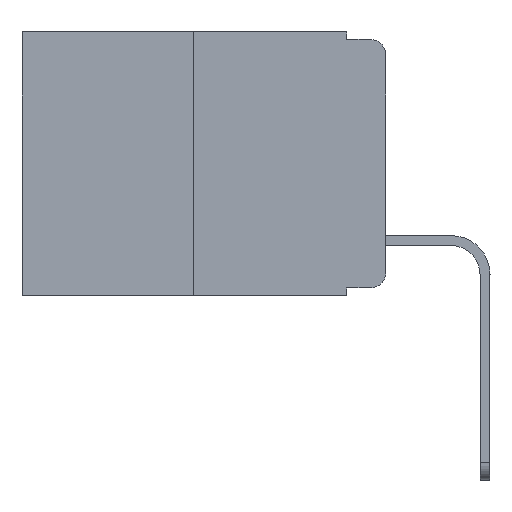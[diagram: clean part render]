
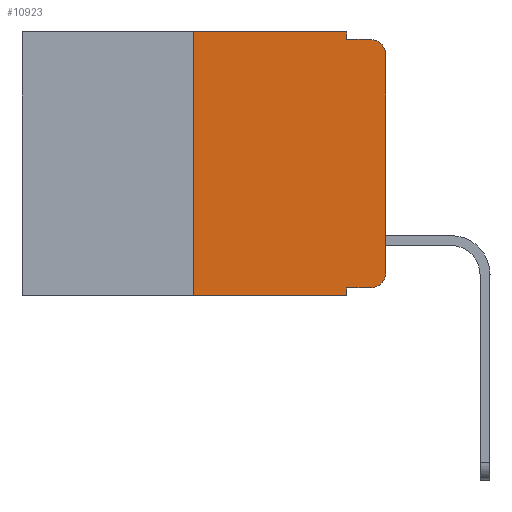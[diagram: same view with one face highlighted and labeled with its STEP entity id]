
A CAD part, left-side view. The second image highlights one B-rep face of the part: STEP entity #10923.
In plain terms, the highlighted planar face has unit normal (-1, 0, 0).
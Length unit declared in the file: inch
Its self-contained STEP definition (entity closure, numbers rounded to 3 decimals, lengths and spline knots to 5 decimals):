
#735 = AXIS2_PLACEMENT_3D ( 'NONE', #8578, #4028, #10306 ) ;
#1139 = ORIENTED_EDGE ( 'NONE', *, *, #16479, .F. ) ;
#1734 = VERTEX_POINT ( 'NONE', #15935 ) ;
#1859 = ORIENTED_EDGE ( 'NONE', *, *, #16016, .T. ) ;
#1916 = VECTOR ( 'NONE', #7416, 39.37008 ) ;
#2189 = EDGE_CURVE ( 'NONE', #13208, #11674, #11388, .T. ) ;
#2305 = VERTEX_POINT ( 'NONE', #10817 ) ;
#2534 = CARTESIAN_POINT ( 'NONE',  ( 0., 0.051, 0. ) ) ;
#2593 = CARTESIAN_POINT ( 'NONE',  ( 0., 0., -0.313 ) ) ;
#2648 = AXIS2_PLACEMENT_3D ( 'NONE', #5903, #4383, #7565 ) ;
#2926 = DIRECTION ( 'NONE',  ( 0., 0., -1. ) ) ;
#3054 = VECTOR ( 'NONE', #14408, 39.37008 ) ;
#3266 = ORIENTED_EDGE ( 'NONE', *, *, #9544, .F. ) ;
#3595 = LINE ( 'NONE', #6675, #12977 ) ;
#4028 = DIRECTION ( 'NONE',  ( -1., 0., 0. ) ) ;
#4291 = DIRECTION ( 'NONE',  ( 0., 0., 1. ) ) ;
#4344 = DIRECTION ( 'NONE',  ( 0., 0., 1. ) ) ;
#4383 = DIRECTION ( 'NONE',  ( -1., 0., 0. ) ) ;
#4398 = ORIENTED_EDGE ( 'NONE', *, *, #7816, .T. ) ;
#5777 = VERTEX_POINT ( 'NONE', #2593 ) ;
#5903 = CARTESIAN_POINT ( 'NONE',  ( 0., 0.02, -0.03 ) ) ;
#6162 = LINE ( 'NONE', #12138, #19454 ) ;
#6201 = FACE_OUTER_BOUND ( 'NONE', #10131, .T. ) ;
#6270 = LINE ( 'NONE', #7984, #3054 ) ;
#6675 = CARTESIAN_POINT ( 'NONE',  ( 0., 0.473, -0.343 ) ) ;
#7071 = EDGE_CURVE ( 'NONE', #1734, #2305, #11300, .T. ) ;
#7093 = LINE ( 'NONE', #2534, #1916 ) ;
#7170 = ORIENTED_EDGE ( 'NONE', *, *, #12953, .T. ) ;
#7213 = CARTESIAN_POINT ( 'NONE',  ( 0., 0.051, -0.01 ) ) ;
#7250 = VERTEX_POINT ( 'NONE', #16782 ) ;
#7416 = DIRECTION ( 'NONE',  ( 0., 0., -1. ) ) ;
#7453 = CARTESIAN_POINT ( 'NONE',  ( 0., 0.25, 0. ) ) ;
#7562 = CARTESIAN_POINT ( 'NONE',  ( 0., 0.02, -0.01 ) ) ;
#7565 = DIRECTION ( 'NONE',  ( 0., 0., -1. ) ) ;
#7729 = AXIS2_PLACEMENT_3D ( 'NONE', #7776, #15755, #9570 ) ;
#7770 = VECTOR ( 'NONE', #2926, 39.37008 ) ;
#7776 = CARTESIAN_POINT ( 'NONE',  ( 0., 0.473, 0. ) ) ;
#7816 = EDGE_CURVE ( 'NONE', #12070, #16384, #11991, .T. ) ;
#7984 = CARTESIAN_POINT ( 'NONE',  ( 0., 0.473, 0. ) ) ;
#8578 = CARTESIAN_POINT ( 'NONE',  ( 0., 0.02, -0.313 ) ) ;
#8615 = CARTESIAN_POINT ( 'NONE',  ( 0., 0.051, -0.333 ) ) ;
#8996 = LINE ( 'NONE', #20204, #7770 ) ;
#9261 = EDGE_CURVE ( 'NONE', #11674, #15779, #6270, .T. ) ;
#9544 = EDGE_CURVE ( 'NONE', #16364, #16384, #17073, .T. ) ;
#9570 = DIRECTION ( 'NONE',  ( 0., 0., -1. ) ) ;
#9854 = ORIENTED_EDGE ( 'NONE', *, *, #7071, .T. ) ;
#10131 = EDGE_LOOP ( 'NONE', ( #17445, #4398, #3266, #1139, #18250, #13309, #1859, #11216, #9854, #7170 ) ) ;
#10306 = DIRECTION ( 'NONE',  ( 0., 0., -1. ) ) ;
#10817 = CARTESIAN_POINT ( 'NONE',  ( 0., 0.02, -0.333 ) ) ;
#10923 = ADVANCED_FACE ( 'NONE', ( #6201 ), #17249, .F. ) ;
#11216 = ORIENTED_EDGE ( 'NONE', *, *, #14319, .F. ) ;
#11300 = LINE ( 'NONE', #8615, #19158 ) ;
#11388 = LINE ( 'NONE', #7453, #20243 ) ;
#11674 = VERTEX_POINT ( 'NONE', #14443 ) ;
#11849 = DIRECTION ( 'NONE',  ( 0., -1., 0. ) ) ;
#11991 = CIRCLE ( 'NONE', #2648, 0.02 ) ;
#12070 = VERTEX_POINT ( 'NONE', #12670 ) ;
#12138 = CARTESIAN_POINT ( 'NONE',  ( 0., 0., 0. ) ) ;
#12398 = VECTOR ( 'NONE', #16691, 39.37008 ) ;
#12449 = CARTESIAN_POINT ( 'NONE',  ( 0., 0.051, 0. ) ) ;
#12670 = CARTESIAN_POINT ( 'NONE',  ( 0., 0., -0.03 ) ) ;
#12953 = EDGE_CURVE ( 'NONE', #2305, #5777, #16983, .T. ) ;
#12977 = VECTOR ( 'NONE', #19248, 39.37008 ) ;
#13043 = EDGE_CURVE ( 'NONE', #5777, #12070, #6162, .T. ) ;
#13208 = VERTEX_POINT ( 'NONE', #18723 ) ;
#13309 = ORIENTED_EDGE ( 'NONE', *, *, #2189, .F. ) ;
#14319 = EDGE_CURVE ( 'NONE', #1734, #7250, #7093, .T. ) ;
#14408 = DIRECTION ( 'NONE',  ( 0., -1., 0. ) ) ;
#14443 = CARTESIAN_POINT ( 'NONE',  ( 0., 0.25, 0. ) ) ;
#15755 = DIRECTION ( 'NONE',  ( 1., 0., 0. ) ) ;
#15779 = VERTEX_POINT ( 'NONE', #12449 ) ;
#15935 = CARTESIAN_POINT ( 'NONE',  ( 0., 0.051, -0.333 ) ) ;
#16016 = EDGE_CURVE ( 'NONE', #13208, #7250, #3595, .T. ) ;
#16364 = VERTEX_POINT ( 'NONE', #16767 ) ;
#16384 = VERTEX_POINT ( 'NONE', #7562 ) ;
#16479 = EDGE_CURVE ( 'NONE', #15779, #16364, #8996, .T. ) ;
#16691 = DIRECTION ( 'NONE',  ( 0., -1., 0. ) ) ;
#16767 = CARTESIAN_POINT ( 'NONE',  ( 0., 0.051, -0.01 ) ) ;
#16782 = CARTESIAN_POINT ( 'NONE',  ( 0., 0.051, -0.343 ) ) ;
#16983 = CIRCLE ( 'NONE', #735, 0.02 ) ;
#17073 = LINE ( 'NONE', #7213, #12398 ) ;
#17249 = PLANE ( 'NONE',  #7729 ) ;
#17445 = ORIENTED_EDGE ( 'NONE', *, *, #13043, .T. ) ;
#18250 = ORIENTED_EDGE ( 'NONE', *, *, #9261, .F. ) ;
#18723 = CARTESIAN_POINT ( 'NONE',  ( 0., 0.25, -0.343 ) ) ;
#19158 = VECTOR ( 'NONE', #11849, 39.37008 ) ;
#19248 = DIRECTION ( 'NONE',  ( 0., -1., 0. ) ) ;
#19454 = VECTOR ( 'NONE', #4291, 39.37008 ) ;
#20204 = CARTESIAN_POINT ( 'NONE',  ( 0., 0.051, 0. ) ) ;
#20243 = VECTOR ( 'NONE', #4344, 39.37008 ) ;
